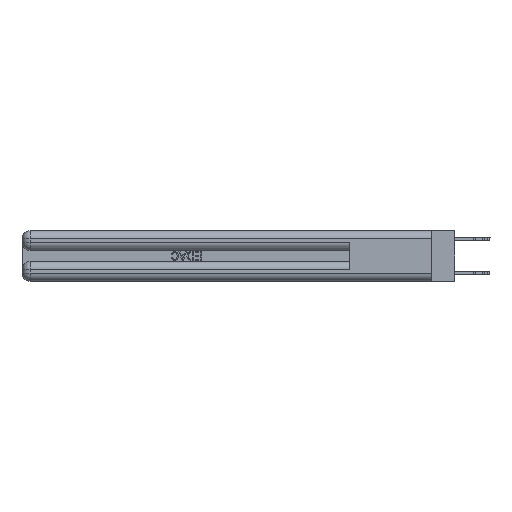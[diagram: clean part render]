
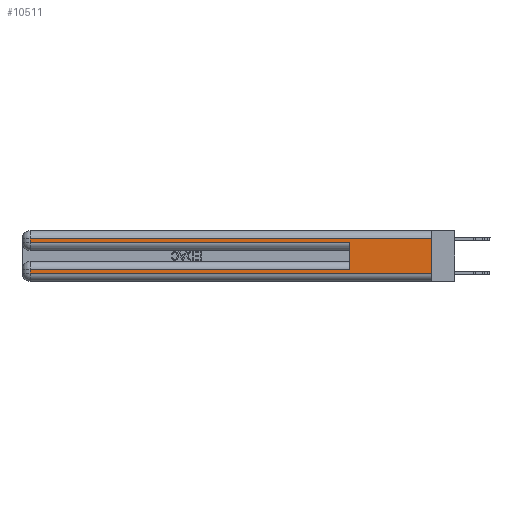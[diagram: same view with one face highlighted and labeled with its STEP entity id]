
A CAD part, left-side view. The second image highlights one B-rep face of the part: STEP entity #10511.
In plain terms, the highlighted planar face has unit normal (-1, 0, 0).
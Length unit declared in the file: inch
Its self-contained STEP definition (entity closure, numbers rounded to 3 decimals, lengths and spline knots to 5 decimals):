
#167 = ORIENTED_EDGE ( 'NONE', *, *, #7889, .T. ) ;
#537 = CARTESIAN_POINT ( 'NONE',  ( 0., 0., 0.37 ) ) ;
#1851 = CARTESIAN_POINT ( 'NONE',  ( 0., 0., 0.085 ) ) ;
#1917 = VERTEX_POINT ( 'NONE', #3372 ) ;
#2413 = CARTESIAN_POINT ( 'NONE',  ( 0., 0., 0.37 ) ) ;
#2872 = EDGE_CURVE ( 'NONE', #13604, #3729, #9507, .T. ) ;
#3129 = LINE ( 'NONE', #13822, #12229 ) ;
#3372 = CARTESIAN_POINT ( 'NONE',  ( 0., 0.6, 0.285 ) ) ;
#3729 = VERTEX_POINT ( 'NONE', #26285 ) ;
#3731 = VECTOR ( 'NONE', #12157, 39.37008 ) ;
#3949 = EDGE_CURVE ( 'NONE', #3729, #14678, #3129, .T. ) ;
#4295 = VERTEX_POINT ( 'NONE', #5069 ) ;
#4935 = DIRECTION ( 'NONE',  ( 0., 0., -1. ) ) ;
#5069 = CARTESIAN_POINT ( 'NONE',  ( 0., 0., 0.31 ) ) ;
#6319 = EDGE_CURVE ( 'NONE', #28941, #1917, #10247, .T. ) ;
#6677 = ORIENTED_EDGE ( 'NONE', *, *, #18392, .F. ) ;
#7040 = DIRECTION ( 'NONE',  ( 0., -1., 0. ) ) ;
#7690 = EDGE_CURVE ( 'NONE', #4295, #25891, #29457, .T. ) ;
#7889 = EDGE_CURVE ( 'NONE', #14678, #25891, #14841, .T. ) ;
#8380 = VECTOR ( 'NONE', #34090, 39.37008 ) ;
#9336 = EDGE_CURVE ( 'NONE', #26286, #28941, #20777, .T. ) ;
#9507 = LINE ( 'NONE', #1851, #8380 ) ;
#9659 = ORIENTED_EDGE ( 'NONE', *, *, #6319, .T. ) ;
#10247 = LINE ( 'NONE', #31427, #24476 ) ;
#10511 = ADVANCED_FACE ( 'NONE', ( #13210 ), #13741, .F. ) ;
#10586 = DIRECTION ( 'NONE',  ( 0., 0., 1. ) ) ;
#11415 = DIRECTION ( 'NONE',  ( 1., 0., 0. ) ) ;
#12119 = ORIENTED_EDGE ( 'NONE', *, *, #9336, .T. ) ;
#12157 = DIRECTION ( 'NONE',  ( 0., -1., 0. ) ) ;
#12229 = VECTOR ( 'NONE', #21987, 39.37008 ) ;
#12324 = ORIENTED_EDGE ( 'NONE', *, *, #3949, .T. ) ;
#13210 = FACE_OUTER_BOUND ( 'NONE', #31476, .T. ) ;
#13269 = DIRECTION ( 'NONE',  ( 0., 0., -1. ) ) ;
#13604 = VERTEX_POINT ( 'NONE', #26812 ) ;
#13741 = PLANE ( 'NONE',  #34051 ) ;
#13822 = CARTESIAN_POINT ( 'NONE',  ( 0., 2.94, 0.37 ) ) ;
#14678 = VERTEX_POINT ( 'NONE', #24886 ) ;
#14841 = LINE ( 'NONE', #20351, #3731 ) ;
#15212 = LINE ( 'NONE', #18066, #21798 ) ;
#18066 = CARTESIAN_POINT ( 'NONE',  ( 0., 0.6, 0.145 ) ) ;
#18392 = EDGE_CURVE ( 'NONE', #13604, #1917, #15212, .T. ) ;
#19225 = VECTOR ( 'NONE', #4935, 39.37008 ) ;
#19574 = ORIENTED_EDGE ( 'NONE', *, *, #7690, .F. ) ;
#20351 = CARTESIAN_POINT ( 'NONE',  ( 0., 0., 0.06 ) ) ;
#20777 = LINE ( 'NONE', #32350, #19225 ) ;
#20786 = EDGE_CURVE ( 'NONE', #4295, #26286, #23838, .T. ) ;
#21516 = DIRECTION ( 'NONE',  ( 0., 1., 0. ) ) ;
#21798 = VECTOR ( 'NONE', #10586, 39.37008 ) ;
#21987 = DIRECTION ( 'NONE',  ( 0., 0., -1. ) ) ;
#23838 = LINE ( 'NONE', #34727, #30387 ) ;
#24476 = VECTOR ( 'NONE', #7040, 39.37008 ) ;
#24520 = CARTESIAN_POINT ( 'NONE',  ( 0., 2.94, 0.31 ) ) ;
#24886 = CARTESIAN_POINT ( 'NONE',  ( 0., 2.94, 0.06 ) ) ;
#25278 = DIRECTION ( 'NONE',  ( 0., 0., -1. ) ) ;
#25891 = VERTEX_POINT ( 'NONE', #29367 ) ;
#26285 = CARTESIAN_POINT ( 'NONE',  ( 0., 2.94, 0.085 ) ) ;
#26286 = VERTEX_POINT ( 'NONE', #24520 ) ;
#26812 = CARTESIAN_POINT ( 'NONE',  ( 0., 0.6, 0.085 ) ) ;
#28941 = VERTEX_POINT ( 'NONE', #33960 ) ;
#28951 = VECTOR ( 'NONE', #13269, 39.37008 ) ;
#29367 = CARTESIAN_POINT ( 'NONE',  ( 0., 0., 0.06 ) ) ;
#29457 = LINE ( 'NONE', #2413, #28951 ) ;
#30387 = VECTOR ( 'NONE', #21516, 39.37008 ) ;
#31427 = CARTESIAN_POINT ( 'NONE',  ( 0., 0., 0.285 ) ) ;
#31476 = EDGE_LOOP ( 'NONE', ( #19574, #34180, #12119, #9659, #6677, #32520, #12324, #167 ) ) ;
#32350 = CARTESIAN_POINT ( 'NONE',  ( 0., 2.94, 0.37 ) ) ;
#32520 = ORIENTED_EDGE ( 'NONE', *, *, #2872, .T. ) ;
#33960 = CARTESIAN_POINT ( 'NONE',  ( 0., 2.94, 0.285 ) ) ;
#34051 = AXIS2_PLACEMENT_3D ( 'NONE', #537, #11415, #25278 ) ;
#34090 = DIRECTION ( 'NONE',  ( 0., 1., 0. ) ) ;
#34180 = ORIENTED_EDGE ( 'NONE', *, *, #20786, .T. ) ;
#34727 = CARTESIAN_POINT ( 'NONE',  ( 0., 0., 0.31 ) ) ;
